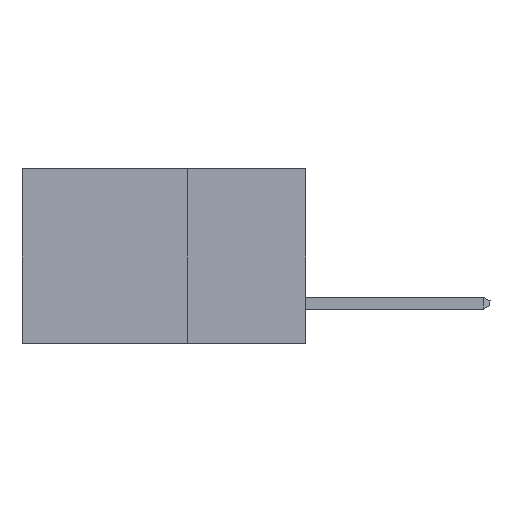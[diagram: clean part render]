
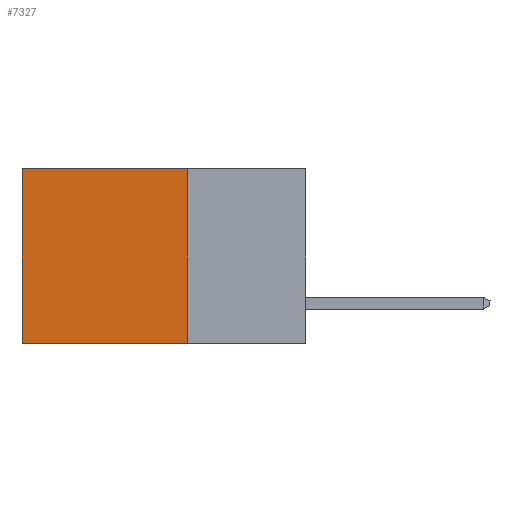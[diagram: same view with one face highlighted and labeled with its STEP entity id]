
A CAD part, left-side view. The second image highlights one B-rep face of the part: STEP entity #7327.
In plain terms, the highlighted planar face has unit normal (-1, 0, 0).
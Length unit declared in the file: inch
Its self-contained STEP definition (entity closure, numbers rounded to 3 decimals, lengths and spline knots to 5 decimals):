
#394 = DIRECTION ( 'NONE',  ( 0., 0., -1. ) ) ;
#736 = VECTOR ( 'NONE', #394, 39.37008 ) ;
#882 = VERTEX_POINT ( 'NONE', #13945 ) ;
#945 = CARTESIAN_POINT ( 'NONE',  ( 0.2615, 0.25, -0.37 ) ) ;
#954 = ORIENTED_EDGE ( 'NONE', *, *, #3494, .T. ) ;
#988 = LINE ( 'NONE', #8682, #1390 ) ;
#1390 = VECTOR ( 'NONE', #12191, 39.37008 ) ;
#1650 = LINE ( 'NONE', #13946, #6775 ) ;
#1660 = ORIENTED_EDGE ( 'NONE', *, *, #10741, .F. ) ;
#1670 = CARTESIAN_POINT ( 'NONE',  ( 0.2615, 0.25, -0.37 ) ) ;
#2071 = DIRECTION ( 'NONE',  ( 0., 0., -1. ) ) ;
#2695 = CARTESIAN_POINT ( 'NONE',  ( 0.2615, 0.6, 0. ) ) ;
#2878 = PLANE ( 'NONE',  #4622 ) ;
#3256 = LINE ( 'NONE', #8158, #3664 ) ;
#3462 = VERTEX_POINT ( 'NONE', #1670 ) ;
#3494 = EDGE_CURVE ( 'NONE', #5790, #8469, #11363, .T. ) ;
#3664 = VECTOR ( 'NONE', #2071, 39.37008 ) ;
#3900 = CARTESIAN_POINT ( 'NONE',  ( 0.2615, 0.6, -0.37 ) ) ;
#4078 = FACE_OUTER_BOUND ( 'NONE', #6212, .T. ) ;
#4622 = AXIS2_PLACEMENT_3D ( 'NONE', #945, #10567, #15352 ) ;
#4971 = CARTESIAN_POINT ( 'NONE',  ( 0.2615, 0.6, -0.37 ) ) ;
#5790 = VERTEX_POINT ( 'NONE', #2695 ) ;
#6212 = EDGE_LOOP ( 'NONE', ( #954, #15663, #1660, #14268 ) ) ;
#6775 = VECTOR ( 'NONE', #11411, 39.37008 ) ;
#7327 = ADVANCED_FACE ( 'NONE', ( #4078 ), #2878, .F. ) ;
#8158 = CARTESIAN_POINT ( 'NONE',  ( 0.2615, 0.25, -0.37 ) ) ;
#8469 = VERTEX_POINT ( 'NONE', #4971 ) ;
#8682 = CARTESIAN_POINT ( 'NONE',  ( 0.2615, 0.25, -0.37 ) ) ;
#10567 = DIRECTION ( 'NONE',  ( 1., 0., 0. ) ) ;
#10741 = EDGE_CURVE ( 'NONE', #882, #3462, #3256, .T. ) ;
#11363 = LINE ( 'NONE', #3900, #736 ) ;
#11411 = DIRECTION ( 'NONE',  ( 0., 1., 0. ) ) ;
#11490 = EDGE_CURVE ( 'NONE', #882, #5790, #1650, .T. ) ;
#12191 = DIRECTION ( 'NONE',  ( 0., 1., 0. ) ) ;
#13108 = EDGE_CURVE ( 'NONE', #3462, #8469, #988, .T. ) ;
#13945 = CARTESIAN_POINT ( 'NONE',  ( 0.2615, 0.25, 0. ) ) ;
#13946 = CARTESIAN_POINT ( 'NONE',  ( 0.2615, 0.25, 0. ) ) ;
#14268 = ORIENTED_EDGE ( 'NONE', *, *, #11490, .T. ) ;
#15352 = DIRECTION ( 'NONE',  ( 0., 0., -1. ) ) ;
#15663 = ORIENTED_EDGE ( 'NONE', *, *, #13108, .F. ) ;
